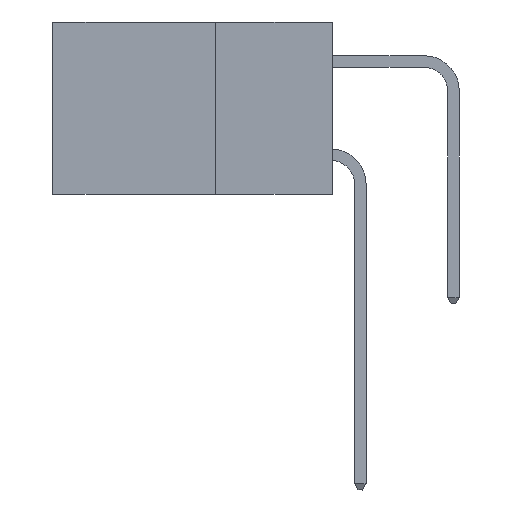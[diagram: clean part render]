
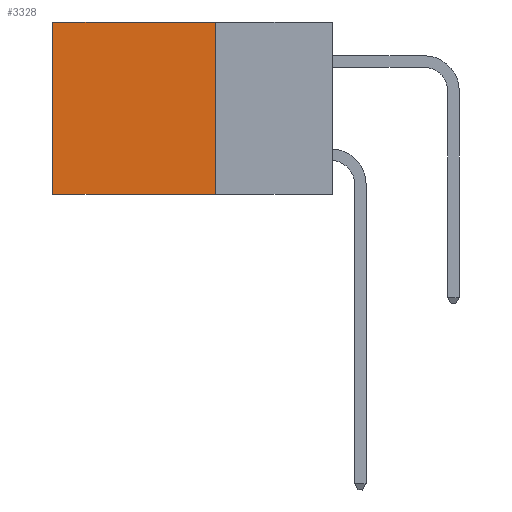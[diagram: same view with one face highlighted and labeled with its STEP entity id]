
A CAD part, left-side view. The second image highlights one B-rep face of the part: STEP entity #3328.
In plain terms, the highlighted planar face has unit normal (-1, 0, 0).
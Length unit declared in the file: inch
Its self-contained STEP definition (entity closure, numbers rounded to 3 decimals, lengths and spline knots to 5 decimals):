
#29 = CARTESIAN_POINT ( 'NONE',  ( 0.298, 0.25, 0. ) ) ;
#404 = VECTOR ( 'NONE', #5876, 39.37008 ) ;
#408 = EDGE_CURVE ( 'NONE', #5156, #7624, #8513, .T. ) ;
#412 = DIRECTION ( 'NONE',  ( 0., 0., -1. ) ) ;
#558 = CARTESIAN_POINT ( 'NONE',  ( 0.298, 0.25, -0.37 ) ) ;
#559 = DIRECTION ( 'NONE',  ( 0., 1., 0. ) ) ;
#649 = LINE ( 'NONE', #6094, #404 ) ;
#1054 = CARTESIAN_POINT ( 'NONE',  ( 0.298, 0.25, 0. ) ) ;
#2731 = ORIENTED_EDGE ( 'NONE', *, *, #5452, .F. ) ;
#3022 = AXIS2_PLACEMENT_3D ( 'NONE', #1054, #7090, #412 ) ;
#3180 = LINE ( 'NONE', #4786, #9924 ) ;
#3328 = ADVANCED_FACE ( 'NONE', ( #4741 ), #5304, .F. ) ;
#4231 = VERTEX_POINT ( 'NONE', #558 ) ;
#4741 = FACE_OUTER_BOUND ( 'NONE', #9732, .T. ) ;
#4756 = ORIENTED_EDGE ( 'NONE', *, *, #10138, .T. ) ;
#4786 = CARTESIAN_POINT ( 'NONE',  ( 0.298, 0.25, -0.37 ) ) ;
#5156 = VERTEX_POINT ( 'NONE', #8550 ) ;
#5217 = VECTOR ( 'NONE', #7708, 39.37008 ) ;
#5304 = PLANE ( 'NONE',  #3022 ) ;
#5452 = EDGE_CURVE ( 'NONE', #4231, #11021, #3180, .T. ) ;
#5856 = ORIENTED_EDGE ( 'NONE', *, *, #408, .T. ) ;
#5876 = DIRECTION ( 'NONE',  ( 0., 0., -1. ) ) ;
#6094 = CARTESIAN_POINT ( 'NONE',  ( 0.298, 0.6, 0. ) ) ;
#6100 = VECTOR ( 'NONE', #559, 39.37008 ) ;
#7090 = DIRECTION ( 'NONE',  ( 1., 0., 0. ) ) ;
#7179 = EDGE_CURVE ( 'NONE', #5156, #4231, #7613, .T. ) ;
#7613 = LINE ( 'NONE', #7970, #5217 ) ;
#7624 = VERTEX_POINT ( 'NONE', #10040 ) ;
#7708 = DIRECTION ( 'NONE',  ( 0., 0., -1. ) ) ;
#7921 = CARTESIAN_POINT ( 'NONE',  ( 0.298, 0.6, -0.37 ) ) ;
#7970 = CARTESIAN_POINT ( 'NONE',  ( 0.298, 0.25, 0. ) ) ;
#8513 = LINE ( 'NONE', #29, #6100 ) ;
#8550 = CARTESIAN_POINT ( 'NONE',  ( 0.298, 0.25, 0. ) ) ;
#8981 = ORIENTED_EDGE ( 'NONE', *, *, #7179, .F. ) ;
#9732 = EDGE_LOOP ( 'NONE', ( #4756, #2731, #8981, #5856 ) ) ;
#9924 = VECTOR ( 'NONE', #10368, 39.37008 ) ;
#10040 = CARTESIAN_POINT ( 'NONE',  ( 0.298, 0.6, 0. ) ) ;
#10138 = EDGE_CURVE ( 'NONE', #7624, #11021, #649, .T. ) ;
#10368 = DIRECTION ( 'NONE',  ( 0., 1., 0. ) ) ;
#11021 = VERTEX_POINT ( 'NONE', #7921 ) ;
